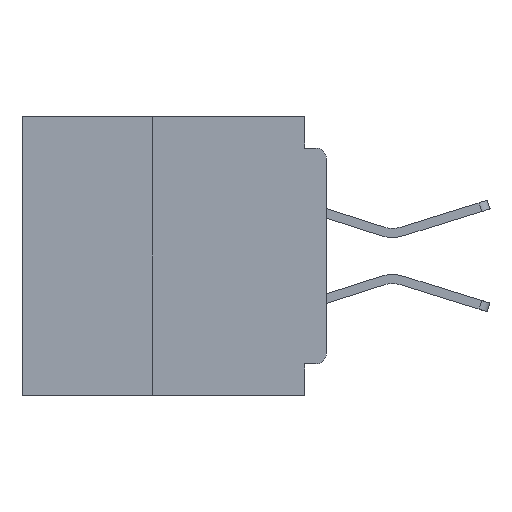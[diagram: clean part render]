
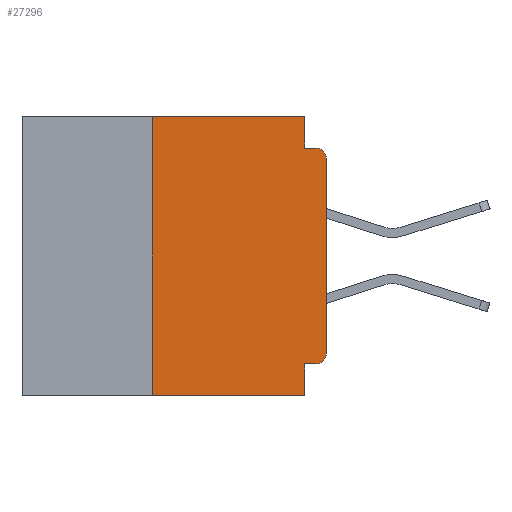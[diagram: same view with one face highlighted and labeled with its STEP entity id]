
A CAD part, left-side view. The second image highlights one B-rep face of the part: STEP entity #27296.
In plain terms, the highlighted planar face has unit normal (-1, 0, 0).
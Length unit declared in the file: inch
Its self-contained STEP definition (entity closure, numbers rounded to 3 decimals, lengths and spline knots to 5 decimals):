
#433 = CARTESIAN_POINT ( 'NONE',  ( 0., 0.015, -0.355 ) ) ;
#637 = DIRECTION ( 'NONE',  ( 0., -1., 0. ) ) ;
#895 = DIRECTION ( 'NONE',  ( -1., 0., 0. ) ) ;
#925 = LINE ( 'NONE', #18201, #29276 ) ;
#2485 = LINE ( 'NONE', #27512, #16986 ) ;
#2551 = ORIENTED_EDGE ( 'NONE', *, *, #16339, .F. ) ;
#3447 = VERTEX_POINT ( 'NONE', #11249 ) ;
#3915 = DIRECTION ( 'NONE',  ( 0., 0., 1. ) ) ;
#3951 = FACE_OUTER_BOUND ( 'NONE', #8110, .T. ) ;
#4277 = ORIENTED_EDGE ( 'NONE', *, *, #21338, .T. ) ;
#5095 = VERTEX_POINT ( 'NONE', #19515 ) ;
#5736 = AXIS2_PLACEMENT_3D ( 'NONE', #22830, #31098, #14563 ) ;
#5807 = VECTOR ( 'NONE', #10114, 39.37008 ) ;
#6016 = CARTESIAN_POINT ( 'NONE',  ( 0., 0.437, 0. ) ) ;
#6078 = ORIENTED_EDGE ( 'NONE', *, *, #26335, .F. ) ;
#6303 = CARTESIAN_POINT ( 'NONE',  ( 0., 0.25, -0.4 ) ) ;
#6314 = CARTESIAN_POINT ( 'NONE',  ( 0., 0., 0. ) ) ;
#6913 = LINE ( 'NONE', #18399, #13703 ) ;
#7328 = EDGE_CURVE ( 'NONE', #3447, #14146, #2485, .T. ) ;
#8110 = EDGE_LOOP ( 'NONE', ( #9890, #4277, #36047, #6078, #2551, #32157, #23857, #10535, #26368, #9384 ) ) ;
#8541 = LINE ( 'NONE', #6016, #22711 ) ;
#8674 = LINE ( 'NONE', #6314, #23707 ) ;
#8689 = EDGE_CURVE ( 'NONE', #29510, #10922, #18663, .T. ) ;
#8930 = DIRECTION ( 'NONE',  ( 0., -1., 0. ) ) ;
#9384 = ORIENTED_EDGE ( 'NONE', *, *, #8689, .T. ) ;
#9890 = ORIENTED_EDGE ( 'NONE', *, *, #13902, .T. ) ;
#10114 = DIRECTION ( 'NONE',  ( 0., 0., -1. ) ) ;
#10535 = ORIENTED_EDGE ( 'NONE', *, *, #7328, .F. ) ;
#10922 = VERTEX_POINT ( 'NONE', #14768 ) ;
#11249 = CARTESIAN_POINT ( 'NONE',  ( 0., 0.031, -0.355 ) ) ;
#13364 = VERTEX_POINT ( 'NONE', #30659 ) ;
#13417 = DIRECTION ( 'NONE',  ( 0., 1., 0. ) ) ;
#13703 = VECTOR ( 'NONE', #3915, 39.37008 ) ;
#13902 = EDGE_CURVE ( 'NONE', #10922, #16575, #8674, .T. ) ;
#14146 = VERTEX_POINT ( 'NONE', #32370 ) ;
#14253 = VECTOR ( 'NONE', #13417, 39.37008 ) ;
#14436 = PLANE ( 'NONE',  #5736 ) ;
#14563 = DIRECTION ( 'NONE',  ( 0., 0., -1. ) ) ;
#14768 = CARTESIAN_POINT ( 'NONE',  ( 0., 0., -0.34 ) ) ;
#15005 = DIRECTION ( 'NONE',  ( -1., 0., 0. ) ) ;
#16339 = EDGE_CURVE ( 'NONE', #13364, #5095, #8541, .T. ) ;
#16575 = VERTEX_POINT ( 'NONE', #34880 ) ;
#16986 = VECTOR ( 'NONE', #28687, 39.37008 ) ;
#17496 = VERTEX_POINT ( 'NONE', #29279 ) ;
#18201 = CARTESIAN_POINT ( 'NONE',  ( 0., 0., -0.045 ) ) ;
#18245 = CARTESIAN_POINT ( 'NONE',  ( 0., 0.015, -0.34 ) ) ;
#18399 = CARTESIAN_POINT ( 'NONE',  ( 0., 0.25, -0.4 ) ) ;
#18663 = CIRCLE ( 'NONE', #33753, 0.015 ) ;
#18920 = VECTOR ( 'NONE', #637, 39.37008 ) ;
#19515 = CARTESIAN_POINT ( 'NONE',  ( 0., 0.031, 0. ) ) ;
#19773 = LINE ( 'NONE', #23502, #18920 ) ;
#20049 = AXIS2_PLACEMENT_3D ( 'NONE', #31530, #15005, #34209 ) ;
#20998 = DIRECTION ( 'NONE',  ( 0., 0., -1. ) ) ;
#21338 = EDGE_CURVE ( 'NONE', #16575, #17496, #27221, .T. ) ;
#21451 = EDGE_CURVE ( 'NONE', #28246, #13364, #6913, .T. ) ;
#22711 = VECTOR ( 'NONE', #8930, 39.37008 ) ;
#22830 = CARTESIAN_POINT ( 'NONE',  ( 0., 0.437, 0. ) ) ;
#23443 = CARTESIAN_POINT ( 'NONE',  ( 0., 0.031, -0.045 ) ) ;
#23502 = CARTESIAN_POINT ( 'NONE',  ( 0., 0.437, -0.4 ) ) ;
#23707 = VECTOR ( 'NONE', #28813, 39.37008 ) ;
#23857 = ORIENTED_EDGE ( 'NONE', *, *, #33481, .T. ) ;
#24131 = CARTESIAN_POINT ( 'NONE',  ( 0., 0.031, 0. ) ) ;
#25537 = VERTEX_POINT ( 'NONE', #23443 ) ;
#26335 = EDGE_CURVE ( 'NONE', #5095, #25537, #35412, .T. ) ;
#26368 = ORIENTED_EDGE ( 'NONE', *, *, #29826, .F. ) ;
#27221 = CIRCLE ( 'NONE', #20049, 0.015 ) ;
#27296 = ADVANCED_FACE ( 'NONE', ( #3951 ), #14436, .F. ) ;
#27512 = CARTESIAN_POINT ( 'NONE',  ( 0., 0.031, -0.4 ) ) ;
#28246 = VERTEX_POINT ( 'NONE', #6303 ) ;
#28687 = DIRECTION ( 'NONE',  ( 0., 0., -1. ) ) ;
#28813 = DIRECTION ( 'NONE',  ( 0., 0., 1. ) ) ;
#29276 = VECTOR ( 'NONE', #34491, 39.37008 ) ;
#29279 = CARTESIAN_POINT ( 'NONE',  ( 0., 0.015, -0.045 ) ) ;
#29510 = VERTEX_POINT ( 'NONE', #433 ) ;
#29826 = EDGE_CURVE ( 'NONE', #29510, #3447, #29846, .T. ) ;
#29846 = LINE ( 'NONE', #30012, #14253 ) ;
#30012 = CARTESIAN_POINT ( 'NONE',  ( 0., 0., -0.355 ) ) ;
#30659 = CARTESIAN_POINT ( 'NONE',  ( 0., 0.25, 0. ) ) ;
#31098 = DIRECTION ( 'NONE',  ( 1., 0., 0. ) ) ;
#31530 = CARTESIAN_POINT ( 'NONE',  ( 0., 0.015, -0.06 ) ) ;
#32157 = ORIENTED_EDGE ( 'NONE', *, *, #21451, .F. ) ;
#32370 = CARTESIAN_POINT ( 'NONE',  ( 0., 0.031, -0.4 ) ) ;
#32372 = EDGE_CURVE ( 'NONE', #25537, #17496, #925, .T. ) ;
#33481 = EDGE_CURVE ( 'NONE', #28246, #14146, #19773, .T. ) ;
#33753 = AXIS2_PLACEMENT_3D ( 'NONE', #18245, #895, #20998 ) ;
#34209 = DIRECTION ( 'NONE',  ( 0., 0., -1. ) ) ;
#34491 = DIRECTION ( 'NONE',  ( 0., -1., 0. ) ) ;
#34880 = CARTESIAN_POINT ( 'NONE',  ( 0., 0., -0.06 ) ) ;
#35412 = LINE ( 'NONE', #24131, #5807 ) ;
#36047 = ORIENTED_EDGE ( 'NONE', *, *, #32372, .F. ) ;
